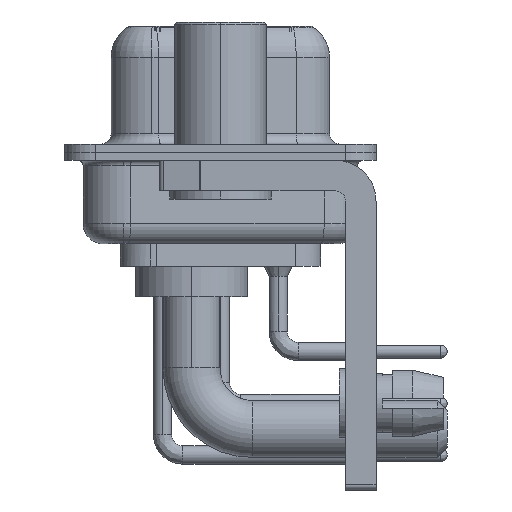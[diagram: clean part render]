
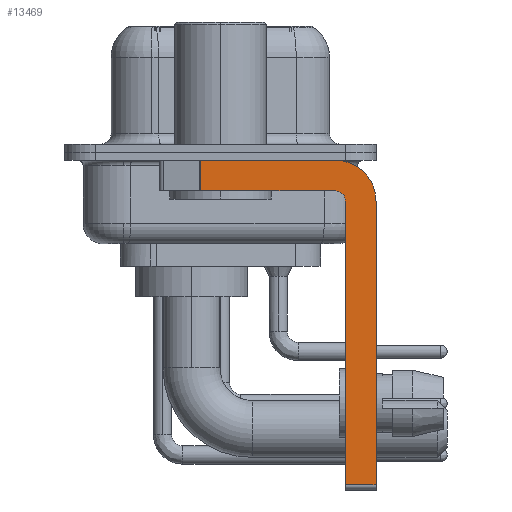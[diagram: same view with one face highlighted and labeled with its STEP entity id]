
A CAD part, left-side view. The second image highlights one B-rep face of the part: STEP entity #13469.
In plain terms, the highlighted planar face has unit normal (-1, 0, 0).
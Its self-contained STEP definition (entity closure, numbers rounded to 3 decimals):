
#296 = ORIENTED_EDGE ( 'NONE', *, *, #30854, .F. ) ;
#1350 = VECTOR ( 'NONE', #22853, 1000. ) ;
#1648 = DIRECTION ( 'NONE',  ( 1., 0., 0. ) ) ;
#2219 = LINE ( 'NONE', #24664, #15977 ) ;
#2376 = ORIENTED_EDGE ( 'NONE', *, *, #10576, .F. ) ;
#2565 = LINE ( 'NONE', #12748, #1350 ) ;
#2884 = CARTESIAN_POINT ( 'NONE',  ( -2.9, -5.65, -0.4 ) ) ;
#2936 = CARTESIAN_POINT ( 'NONE',  ( -2.9, -6.15, -16.6 ) ) ;
#3313 = VECTOR ( 'NONE', #12304, 1000. ) ;
#3441 = CARTESIAN_POINT ( 'NONE',  ( -2.9, 0.978, -1.9 ) ) ;
#3972 = AXIS2_PLACEMENT_3D ( 'NONE', #15357, #15195, #7551 ) ;
#4027 = VERTEX_POINT ( 'NONE', #24469 ) ;
#4165 = ORIENTED_EDGE ( 'NONE', *, *, #5752, .T. ) ;
#4208 = DIRECTION ( 'NONE',  ( 0., 0., 1. ) ) ;
#4290 = VERTEX_POINT ( 'NONE', #28548 ) ;
#4632 = EDGE_CURVE ( 'NONE', #20691, #11660, #27506, .T. ) ;
#4638 = CARTESIAN_POINT ( 'NONE',  ( -2.9, -5.65, -16.35 ) ) ;
#4782 = DIRECTION ( 'NONE',  ( 0., 0., 1. ) ) ;
#4971 = EDGE_CURVE ( 'NONE', #11660, #31135, #24132, .T. ) ;
#5752 = EDGE_CURVE ( 'NONE', #20691, #31309, #18956, .T. ) ;
#6487 = CARTESIAN_POINT ( 'NONE',  ( -2.9, 0.978, -1.9 ) ) ;
#6577 = AXIS2_PLACEMENT_3D ( 'NONE', #9060, #19838, #4208 ) ;
#7551 = DIRECTION ( 'NONE',  ( 0., 0., -1. ) ) ;
#8124 = LINE ( 'NONE', #2936, #12599 ) ;
#9060 = CARTESIAN_POINT ( 'NONE',  ( -2.9, -5.65, -2.4 ) ) ;
#9776 = VECTOR ( 'NONE', #28009, 1000. ) ;
#10239 = CARTESIAN_POINT ( 'NONE',  ( -2.9, 3., -0.4 ) ) ;
#10309 = ORIENTED_EDGE ( 'NONE', *, *, #4632, .F. ) ;
#10576 = EDGE_CURVE ( 'NONE', #31135, #4290, #2219, .T. ) ;
#11660 = VERTEX_POINT ( 'NONE', #2884 ) ;
#11675 = DIRECTION ( 'NONE',  ( 0., 0., -1. ) ) ;
#12304 = DIRECTION ( 'NONE',  ( 0., -1., 0. ) ) ;
#12599 = VECTOR ( 'NONE', #4782, 1000. ) ;
#12748 = CARTESIAN_POINT ( 'NONE',  ( -2.9, -5.65, -1.9 ) ) ;
#12943 = VERTEX_POINT ( 'NONE', #31651 ) ;
#13160 = VERTEX_POINT ( 'NONE', #27458 ) ;
#13469 = ADVANCED_FACE ( 'NONE', ( #19632 ), #24110, .F. ) ;
#14302 = DIRECTION ( 'NONE',  ( 0., 0., -1. ) ) ;
#14484 = EDGE_CURVE ( 'NONE', #12943, #13160, #25642, .T. ) ;
#15195 = DIRECTION ( 'NONE',  ( 1., 0., 0. ) ) ;
#15357 = CARTESIAN_POINT ( 'NONE',  ( -2.9, -5.65, -2.4 ) ) ;
#15977 = VECTOR ( 'NONE', #32651, 1000. ) ;
#16294 = EDGE_LOOP ( 'NONE', ( #10309, #4165, #296, #21804, #24547, #18515, #2376, #32466 ) ) ;
#17912 = CARTESIAN_POINT ( 'NONE',  ( -2.9, -7.65, -2.4 ) ) ;
#18515 = ORIENTED_EDGE ( 'NONE', *, *, #29238, .T. ) ;
#18956 = LINE ( 'NONE', #6487, #19422 ) ;
#18982 = CARTESIAN_POINT ( 'NONE',  ( -2.9, 0.978, -0.4 ) ) ;
#19304 = CARTESIAN_POINT ( 'NONE',  ( -2.9, -5.65, -2.4 ) ) ;
#19422 = VECTOR ( 'NONE', #14302, 1000. ) ;
#19632 = FACE_OUTER_BOUND ( 'NONE', #16294, .T. ) ;
#19838 = DIRECTION ( 'NONE',  ( -1., 0., 0. ) ) ;
#20691 = VERTEX_POINT ( 'NONE', #18982 ) ;
#21563 = EDGE_CURVE ( 'NONE', #4027, #12943, #8124, .T. ) ;
#21804 = ORIENTED_EDGE ( 'NONE', *, *, #14484, .F. ) ;
#22853 = DIRECTION ( 'NONE',  ( 0., 1., 0. ) ) ;
#24110 = PLANE ( 'NONE',  #30355 ) ;
#24132 = CIRCLE ( 'NONE', #3972, 2. ) ;
#24469 = CARTESIAN_POINT ( 'NONE',  ( -2.9, -6.15, -16.35 ) ) ;
#24547 = ORIENTED_EDGE ( 'NONE', *, *, #21563, .F. ) ;
#24664 = CARTESIAN_POINT ( 'NONE',  ( -2.9, -7.65, -2.4 ) ) ;
#24901 = LINE ( 'NONE', #4638, #3313 ) ;
#25642 = CIRCLE ( 'NONE', #6577, 0.5 ) ;
#27458 = CARTESIAN_POINT ( 'NONE',  ( -2.9, -5.65, -1.9 ) ) ;
#27506 = LINE ( 'NONE', #10239, #9776 ) ;
#28009 = DIRECTION ( 'NONE',  ( 0., -1., 0. ) ) ;
#28548 = CARTESIAN_POINT ( 'NONE',  ( -2.9, -7.65, -16.35 ) ) ;
#29238 = EDGE_CURVE ( 'NONE', #4027, #4290, #24901, .T. ) ;
#30355 = AXIS2_PLACEMENT_3D ( 'NONE', #19304, #1648, #11675 ) ;
#30854 = EDGE_CURVE ( 'NONE', #13160, #31309, #2565, .T. ) ;
#31135 = VERTEX_POINT ( 'NONE', #17912 ) ;
#31309 = VERTEX_POINT ( 'NONE', #3441 ) ;
#31651 = CARTESIAN_POINT ( 'NONE',  ( -2.9, -6.15, -2.4 ) ) ;
#32466 = ORIENTED_EDGE ( 'NONE', *, *, #4971, .F. ) ;
#32651 = DIRECTION ( 'NONE',  ( 0., 0., -1. ) ) ;
